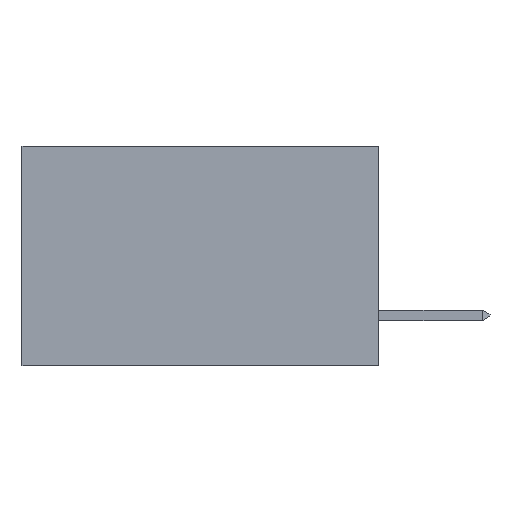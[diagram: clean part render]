
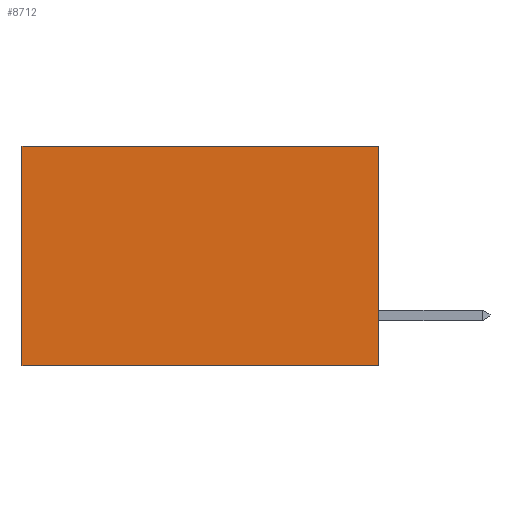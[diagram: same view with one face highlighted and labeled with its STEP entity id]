
A CAD part, left-side view. The second image highlights one B-rep face of the part: STEP entity #8712.
In plain terms, the highlighted planar face has unit normal (-1, 0, 0).
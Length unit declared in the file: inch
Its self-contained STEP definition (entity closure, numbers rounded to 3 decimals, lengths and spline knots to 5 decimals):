
#295 = EDGE_CURVE ( 'NONE', #2963, #6461, #8246, .T. ) ;
#412 = VECTOR ( 'NONE', #7824, 39.37008 ) ;
#431 = CARTESIAN_POINT ( 'NONE',  ( 0.2615, 0., 0. ) ) ;
#560 = DIRECTION ( 'NONE',  ( 0., 0., -1. ) ) ;
#1289 = VECTOR ( 'NONE', #3812, 39.37008 ) ;
#1375 = EDGE_CURVE ( 'NONE', #2963, #7456, #3110, .T. ) ;
#1669 = CARTESIAN_POINT ( 'NONE',  ( 0.2615, 0., -0.37 ) ) ;
#1712 = CARTESIAN_POINT ( 'NONE',  ( 0.2615, 0.6, 0. ) ) ;
#1779 = CARTESIAN_POINT ( 'NONE',  ( 0.2615, 0., 0. ) ) ;
#1948 = EDGE_CURVE ( 'NONE', #6461, #4689, #8463, .T. ) ;
#2029 = DIRECTION ( 'NONE',  ( 1., 0., 0. ) ) ;
#2455 = DIRECTION ( 'NONE',  ( 0., 0., -1. ) ) ;
#2567 = ORIENTED_EDGE ( 'NONE', *, *, #295, .T. ) ;
#2885 = ORIENTED_EDGE ( 'NONE', *, *, #1948, .T. ) ;
#2963 = VERTEX_POINT ( 'NONE', #431 ) ;
#3077 = VECTOR ( 'NONE', #2455, 39.37008 ) ;
#3110 = LINE ( 'NONE', #6793, #3077 ) ;
#3318 = AXIS2_PLACEMENT_3D ( 'NONE', #5000, #2029, #560 ) ;
#3812 = DIRECTION ( 'NONE',  ( 0., 1., 0. ) ) ;
#3977 = ORIENTED_EDGE ( 'NONE', *, *, #7886, .F. ) ;
#4468 = CARTESIAN_POINT ( 'NONE',  ( 0.2615, 0., -0.37 ) ) ;
#4544 = LINE ( 'NONE', #1669, #1289 ) ;
#4689 = VERTEX_POINT ( 'NONE', #9099 ) ;
#4742 = DIRECTION ( 'NONE',  ( 0., 1., 0. ) ) ;
#4777 = CARTESIAN_POINT ( 'NONE',  ( 0.2615, 0.6, -0.37 ) ) ;
#5000 = CARTESIAN_POINT ( 'NONE',  ( 0.2615, 0., -0.37 ) ) ;
#6461 = VERTEX_POINT ( 'NONE', #1712 ) ;
#6793 = CARTESIAN_POINT ( 'NONE',  ( 0.2615, 0., -0.37 ) ) ;
#6911 = ORIENTED_EDGE ( 'NONE', *, *, #1375, .F. ) ;
#7456 = VERTEX_POINT ( 'NONE', #4468 ) ;
#7824 = DIRECTION ( 'NONE',  ( 0., 0., -1. ) ) ;
#7886 = EDGE_CURVE ( 'NONE', #7456, #4689, #4544, .T. ) ;
#8246 = LINE ( 'NONE', #1779, #9242 ) ;
#8463 = LINE ( 'NONE', #4777, #412 ) ;
#8686 = PLANE ( 'NONE',  #3318 ) ;
#8712 = ADVANCED_FACE ( 'NONE', ( #9524 ), #8686, .F. ) ;
#8756 = EDGE_LOOP ( 'NONE', ( #2885, #3977, #6911, #2567 ) ) ;
#9099 = CARTESIAN_POINT ( 'NONE',  ( 0.2615, 0.6, -0.37 ) ) ;
#9242 = VECTOR ( 'NONE', #4742, 39.37008 ) ;
#9524 = FACE_OUTER_BOUND ( 'NONE', #8756, .T. ) ;
